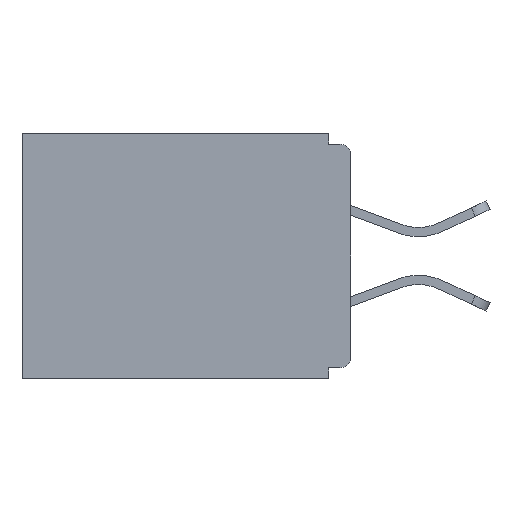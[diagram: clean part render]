
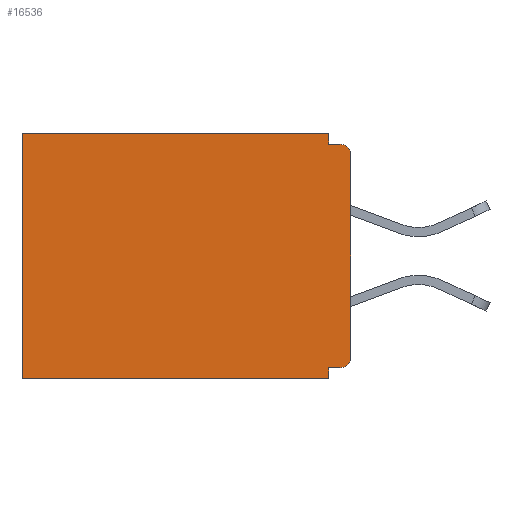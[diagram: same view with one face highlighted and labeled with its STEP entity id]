
A CAD part, left-side view. The second image highlights one B-rep face of the part: STEP entity #16536.
In plain terms, the highlighted planar face has unit normal (-1, 0, 0).
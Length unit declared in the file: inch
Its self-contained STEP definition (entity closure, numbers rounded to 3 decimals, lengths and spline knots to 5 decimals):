
#302 = CARTESIAN_POINT ( 'NONE',  ( 0.298, 0., 0. ) ) ;
#358 = ORIENTED_EDGE ( 'NONE', *, *, #22464, .F. ) ;
#387 = EDGE_CURVE ( 'NONE', #20209, #723, #12396, .T. ) ;
#555 = EDGE_CURVE ( 'NONE', #22853, #13491, #21268, .T. ) ;
#723 = VERTEX_POINT ( 'NONE', #9746 ) ;
#1163 = ORIENTED_EDGE ( 'NONE', *, *, #15754, .F. ) ;
#1180 = EDGE_LOOP ( 'NONE', ( #22773, #10646, #358, #3518, #24303, #21677, #1163, #3997, #26147, #16656 ) ) ;
#1397 = CARTESIAN_POINT ( 'NONE',  ( 0.298, 0.46, 0. ) ) ;
#1956 = VECTOR ( 'NONE', #21081, 39.37008 ) ;
#2063 = VECTOR ( 'NONE', #2403, 39.37008 ) ;
#2403 = DIRECTION ( 'NONE',  ( 0., 0., -1. ) ) ;
#2525 = DIRECTION ( 'NONE',  ( 0., 0., -1. ) ) ;
#2970 = VECTOR ( 'NONE', #13428, 39.37008 ) ;
#3339 = VERTEX_POINT ( 'NONE', #19189 ) ;
#3348 = LINE ( 'NONE', #23441, #11865 ) ;
#3517 = EDGE_CURVE ( 'NONE', #18824, #13491, #3348, .T. ) ;
#3518 = ORIENTED_EDGE ( 'NONE', *, *, #10441, .T. ) ;
#3997 = ORIENTED_EDGE ( 'NONE', *, *, #10235, .F. ) ;
#4249 = CARTESIAN_POINT ( 'NONE',  ( 0.298, 0.031, -0.343 ) ) ;
#4623 = VERTEX_POINT ( 'NONE', #26671 ) ;
#5236 = PLANE ( 'NONE',  #16638 ) ;
#5304 = LINE ( 'NONE', #15654, #6922 ) ;
#5496 = DIRECTION ( 'NONE',  ( 0., 0., -1. ) ) ;
#5766 = FACE_OUTER_BOUND ( 'NONE', #1180, .T. ) ;
#6128 = DIRECTION ( 'NONE',  ( 0., -1., 0. ) ) ;
#6509 = CIRCLE ( 'NONE', #7875, 0.015 ) ;
#6553 = VERTEX_POINT ( 'NONE', #19211 ) ;
#6896 = VECTOR ( 'NONE', #20854, 39.37008 ) ;
#6922 = VECTOR ( 'NONE', #17755, 39.37008 ) ;
#7875 = AXIS2_PLACEMENT_3D ( 'NONE', #25957, #17777, #21644 ) ;
#8475 = CARTESIAN_POINT ( 'NONE',  ( 0.298, 0.015, -0.03 ) ) ;
#8565 = DIRECTION ( 'NONE',  ( -1., 0., 0. ) ) ;
#8912 = CARTESIAN_POINT ( 'NONE',  ( 0.298, 0.031, 0. ) ) ;
#8943 = LINE ( 'NONE', #302, #2063 ) ;
#9016 = CARTESIAN_POINT ( 'NONE',  ( 0.298, 0., -0.343 ) ) ;
#9440 = VERTEX_POINT ( 'NONE', #8912 ) ;
#9746 = CARTESIAN_POINT ( 'NONE',  ( 0.298, 0.015, -0.015 ) ) ;
#10235 = EDGE_CURVE ( 'NONE', #10509, #6553, #12499, .T. ) ;
#10441 = EDGE_CURVE ( 'NONE', #9440, #18824, #15104, .T. ) ;
#10498 = CARTESIAN_POINT ( 'NONE',  ( 0.298, 0., -0.328 ) ) ;
#10509 = VERTEX_POINT ( 'NONE', #19616 ) ;
#10646 = ORIENTED_EDGE ( 'NONE', *, *, #20199, .F. ) ;
#11865 = VECTOR ( 'NONE', #2525, 39.37008 ) ;
#11980 = EDGE_CURVE ( 'NONE', #10509, #3339, #6509, .T. ) ;
#12188 = CARTESIAN_POINT ( 'NONE',  ( 0.298, 0.031, -0.343 ) ) ;
#12396 = CIRCLE ( 'NONE', #24005, 0.015 ) ;
#12499 = LINE ( 'NONE', #10498, #6896 ) ;
#12760 = VECTOR ( 'NONE', #12900, 39.37008 ) ;
#12900 = DIRECTION ( 'NONE',  ( 0., 1., 0. ) ) ;
#12953 = CARTESIAN_POINT ( 'NONE',  ( 0.298, 0.46, -0.343 ) ) ;
#13428 = DIRECTION ( 'NONE',  ( 0., 1., 0. ) ) ;
#13491 = VERTEX_POINT ( 'NONE', #12953 ) ;
#13784 = VECTOR ( 'NONE', #6128, 39.37008 ) ;
#14320 = CARTESIAN_POINT ( 'NONE',  ( 0.298, 0., -0.03 ) ) ;
#15104 = LINE ( 'NONE', #26071, #2970 ) ;
#15654 = CARTESIAN_POINT ( 'NONE',  ( 0.298, 0.031, -0.343 ) ) ;
#15679 = CARTESIAN_POINT ( 'NONE',  ( 0.298, 0., 0. ) ) ;
#15754 = EDGE_CURVE ( 'NONE', #6553, #22853, #5304, .T. ) ;
#16536 = ADVANCED_FACE ( 'NONE', ( #5766 ), #5236, .F. ) ;
#16638 = AXIS2_PLACEMENT_3D ( 'NONE', #15679, #17782, #5496 ) ;
#16656 = ORIENTED_EDGE ( 'NONE', *, *, #18138, .F. ) ;
#16776 = CARTESIAN_POINT ( 'NONE',  ( 0.298, 0., -0.015 ) ) ;
#17755 = DIRECTION ( 'NONE',  ( 0., 0., -1. ) ) ;
#17777 = DIRECTION ( 'NONE',  ( -1., 0., 0. ) ) ;
#17782 = DIRECTION ( 'NONE',  ( 1., 0., 0. ) ) ;
#18138 = EDGE_CURVE ( 'NONE', #20209, #3339, #8943, .T. ) ;
#18375 = LINE ( 'NONE', #16776, #13784 ) ;
#18824 = VERTEX_POINT ( 'NONE', #1397 ) ;
#19189 = CARTESIAN_POINT ( 'NONE',  ( 0.298, 0., -0.313 ) ) ;
#19211 = CARTESIAN_POINT ( 'NONE',  ( 0.298, 0.031, -0.328 ) ) ;
#19616 = CARTESIAN_POINT ( 'NONE',  ( 0.298, 0.015, -0.328 ) ) ;
#20199 = EDGE_CURVE ( 'NONE', #4623, #723, #18375, .T. ) ;
#20209 = VERTEX_POINT ( 'NONE', #14320 ) ;
#20854 = DIRECTION ( 'NONE',  ( 0., 1., 0. ) ) ;
#21081 = DIRECTION ( 'NONE',  ( 0., 0., -1. ) ) ;
#21268 = LINE ( 'NONE', #9016, #12760 ) ;
#21644 = DIRECTION ( 'NONE',  ( 0., 0., -1. ) ) ;
#21677 = ORIENTED_EDGE ( 'NONE', *, *, #555, .F. ) ;
#22464 = EDGE_CURVE ( 'NONE', #9440, #4623, #26895, .T. ) ;
#22773 = ORIENTED_EDGE ( 'NONE', *, *, #387, .T. ) ;
#22853 = VERTEX_POINT ( 'NONE', #4249 ) ;
#23245 = DIRECTION ( 'NONE',  ( 0., 0., -1. ) ) ;
#23441 = CARTESIAN_POINT ( 'NONE',  ( 0.298, 0.46, 0. ) ) ;
#24005 = AXIS2_PLACEMENT_3D ( 'NONE', #8475, #8565, #23245 ) ;
#24303 = ORIENTED_EDGE ( 'NONE', *, *, #3517, .T. ) ;
#25957 = CARTESIAN_POINT ( 'NONE',  ( 0.298, 0.015, -0.313 ) ) ;
#26071 = CARTESIAN_POINT ( 'NONE',  ( 0.298, 0., 0. ) ) ;
#26147 = ORIENTED_EDGE ( 'NONE', *, *, #11980, .T. ) ;
#26671 = CARTESIAN_POINT ( 'NONE',  ( 0.298, 0.031, -0.015 ) ) ;
#26895 = LINE ( 'NONE', #12188, #1956 ) ;
